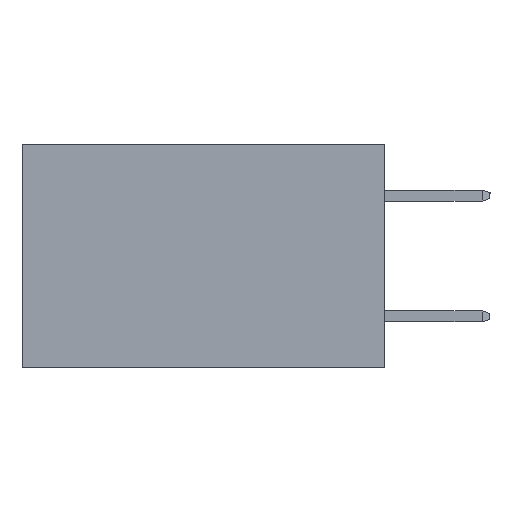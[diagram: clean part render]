
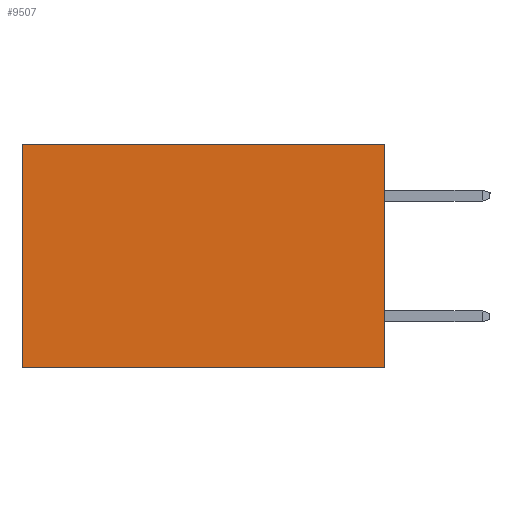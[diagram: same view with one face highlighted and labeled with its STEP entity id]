
A CAD part, left-side view. The second image highlights one B-rep face of the part: STEP entity #9507.
In plain terms, the highlighted planar face has unit normal (-1, 0, 0).
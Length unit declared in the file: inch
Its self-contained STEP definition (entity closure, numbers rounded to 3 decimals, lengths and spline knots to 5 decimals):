
#991 = CARTESIAN_POINT ( 'NONE',  ( 0.2615, 0., 0. ) ) ;
#1335 = VECTOR ( 'NONE', #5342, 39.37008 ) ;
#1648 = FACE_OUTER_BOUND ( 'NONE', #19456, .T. ) ;
#1881 = DIRECTION ( 'NONE',  ( 0., 0., -1. ) ) ;
#2759 = VECTOR ( 'NONE', #6870, 39.37008 ) ;
#3616 = CARTESIAN_POINT ( 'NONE',  ( 0.2615, 0., -0.37 ) ) ;
#3882 = AXIS2_PLACEMENT_3D ( 'NONE', #3616, #15825, #1881 ) ;
#4273 = ORIENTED_EDGE ( 'NONE', *, *, #20540, .F. ) ;
#5065 = VERTEX_POINT ( 'NONE', #991 ) ;
#5342 = DIRECTION ( 'NONE',  ( 0., 0., -1. ) ) ;
#6645 = EDGE_CURVE ( 'NONE', #16476, #13694, #14359, .T. ) ;
#6870 = DIRECTION ( 'NONE',  ( 0., 1., 0. ) ) ;
#8933 = CARTESIAN_POINT ( 'NONE',  ( 0.2615, 0.6, -0.37 ) ) ;
#9017 = PLANE ( 'NONE',  #3882 ) ;
#9507 = ADVANCED_FACE ( 'NONE', ( #1648 ), #9017, .F. ) ;
#9846 = VECTOR ( 'NONE', #13580, 39.37008 ) ;
#10310 = LINE ( 'NONE', #20686, #2759 ) ;
#11408 = CARTESIAN_POINT ( 'NONE',  ( 0.2615, 0.6, -0.37 ) ) ;
#12517 = VERTEX_POINT ( 'NONE', #18762 ) ;
#13201 = CARTESIAN_POINT ( 'NONE',  ( 0.2615, 0.6, 0. ) ) ;
#13245 = LINE ( 'NONE', #14961, #9846 ) ;
#13580 = DIRECTION ( 'NONE',  ( 0., 1., 0. ) ) ;
#13694 = VERTEX_POINT ( 'NONE', #11408 ) ;
#14003 = CARTESIAN_POINT ( 'NONE',  ( 0.2615, 0., -0.37 ) ) ;
#14359 = LINE ( 'NONE', #8933, #20667 ) ;
#14961 = CARTESIAN_POINT ( 'NONE',  ( 0.2615, 0., -0.37 ) ) ;
#15825 = DIRECTION ( 'NONE',  ( 1., 0., 0. ) ) ;
#16118 = EDGE_CURVE ( 'NONE', #5065, #16476, #10310, .T. ) ;
#16476 = VERTEX_POINT ( 'NONE', #13201 ) ;
#17444 = DIRECTION ( 'NONE',  ( 0., 0., -1. ) ) ;
#17652 = LINE ( 'NONE', #14003, #1335 ) ;
#18018 = EDGE_CURVE ( 'NONE', #5065, #12517, #17652, .T. ) ;
#18762 = CARTESIAN_POINT ( 'NONE',  ( 0.2615, 0., -0.37 ) ) ;
#18973 = ORIENTED_EDGE ( 'NONE', *, *, #18018, .F. ) ;
#19456 = EDGE_LOOP ( 'NONE', ( #21842, #4273, #18973, #21223 ) ) ;
#20540 = EDGE_CURVE ( 'NONE', #12517, #13694, #13245, .T. ) ;
#20667 = VECTOR ( 'NONE', #17444, 39.37008 ) ;
#20686 = CARTESIAN_POINT ( 'NONE',  ( 0.2615, 0., 0. ) ) ;
#21223 = ORIENTED_EDGE ( 'NONE', *, *, #16118, .T. ) ;
#21842 = ORIENTED_EDGE ( 'NONE', *, *, #6645, .T. ) ;
